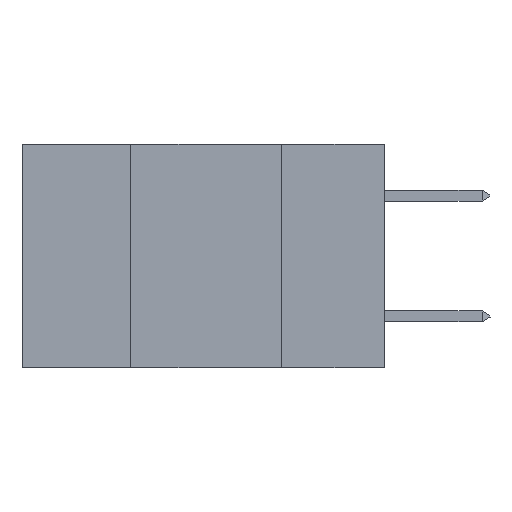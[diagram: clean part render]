
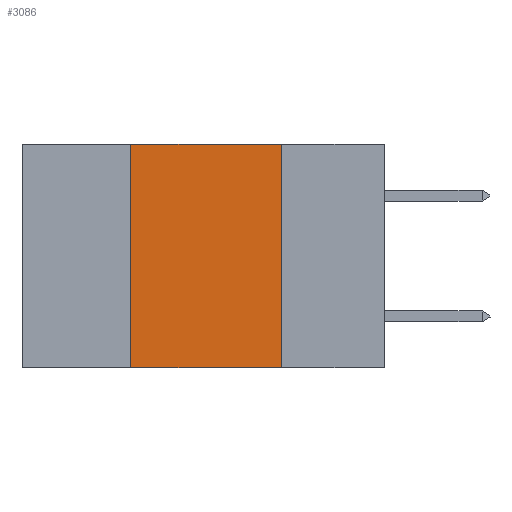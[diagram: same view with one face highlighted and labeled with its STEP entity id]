
A CAD part, left-side view. The second image highlights one B-rep face of the part: STEP entity #3086.
In plain terms, the highlighted planar face has unit normal (-1, 0, 0).
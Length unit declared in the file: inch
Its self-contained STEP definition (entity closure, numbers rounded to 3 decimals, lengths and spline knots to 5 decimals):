
#630 = DIRECTION ( 'NONE',  ( 0., -1., 0. ) ) ;
#1767 = VECTOR ( 'NONE', #7915, 39.37008 ) ;
#1798 = VERTEX_POINT ( 'NONE', #7808 ) ;
#2828 = DIRECTION ( 'NONE',  ( 1., 0., 0. ) ) ;
#3015 = DIRECTION ( 'NONE',  ( 0., 0., -1. ) ) ;
#3086 = ADVANCED_FACE ( 'NONE', ( #18993 ), #9448, .F. ) ;
#3419 = VECTOR ( 'NONE', #13541, 39.37008 ) ;
#4600 = DIRECTION ( 'NONE',  ( 0., 0., -1. ) ) ;
#4651 = ORIENTED_EDGE ( 'NONE', *, *, #18419, .F. ) ;
#6130 = CARTESIAN_POINT ( 'NONE',  ( 0., 0.42, 0. ) ) ;
#6317 = CARTESIAN_POINT ( 'NONE',  ( 0., 0.6, 0. ) ) ;
#7275 = CARTESIAN_POINT ( 'NONE',  ( 0., 0.17, 0. ) ) ;
#7615 = VECTOR ( 'NONE', #3015, 39.37008 ) ;
#7630 = CARTESIAN_POINT ( 'NONE',  ( 0., 0.6, -0.37 ) ) ;
#7808 = CARTESIAN_POINT ( 'NONE',  ( 0., 0.17, -0.37 ) ) ;
#7915 = DIRECTION ( 'NONE',  ( 0., 0., 1. ) ) ;
#8720 = LINE ( 'NONE', #6317, #3419 ) ;
#8760 = CARTESIAN_POINT ( 'NONE',  ( 0., 0.42, 0. ) ) ;
#9046 = VECTOR ( 'NONE', #630, 39.37008 ) ;
#9254 = ORIENTED_EDGE ( 'NONE', *, *, #11481, .F. ) ;
#9448 = PLANE ( 'NONE',  #18867 ) ;
#10674 = ORIENTED_EDGE ( 'NONE', *, *, #18460, .F. ) ;
#10702 = EDGE_CURVE ( 'NONE', #20300, #1798, #13782, .T. ) ;
#11481 = EDGE_CURVE ( 'NONE', #20300, #19230, #15956, .T. ) ;
#11793 = LINE ( 'NONE', #13689, #7615 ) ;
#13541 = DIRECTION ( 'NONE',  ( 0., -1., 0. ) ) ;
#13689 = CARTESIAN_POINT ( 'NONE',  ( 0., 0.17, 0. ) ) ;
#13782 = LINE ( 'NONE', #7630, #9046 ) ;
#15010 = EDGE_LOOP ( 'NONE', ( #10674, #4651, #9254, #20568 ) ) ;
#15956 = LINE ( 'NONE', #6130, #1767 ) ;
#18419 = EDGE_CURVE ( 'NONE', #19230, #20940, #8720, .T. ) ;
#18460 = EDGE_CURVE ( 'NONE', #20940, #1798, #11793, .T. ) ;
#18867 = AXIS2_PLACEMENT_3D ( 'NONE', #18992, #2828, #4600 ) ;
#18992 = CARTESIAN_POINT ( 'NONE',  ( 0., 0.6, 0. ) ) ;
#18993 = FACE_OUTER_BOUND ( 'NONE', #15010, .T. ) ;
#19230 = VERTEX_POINT ( 'NONE', #8760 ) ;
#20300 = VERTEX_POINT ( 'NONE', #22311 ) ;
#20568 = ORIENTED_EDGE ( 'NONE', *, *, #10702, .T. ) ;
#20940 = VERTEX_POINT ( 'NONE', #7275 ) ;
#22311 = CARTESIAN_POINT ( 'NONE',  ( 0., 0.42, -0.37 ) ) ;
